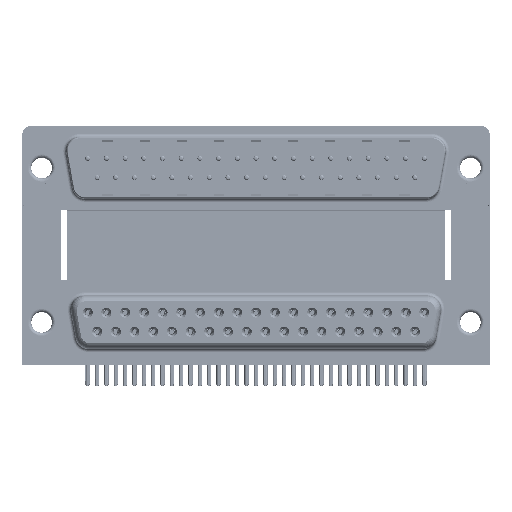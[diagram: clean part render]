
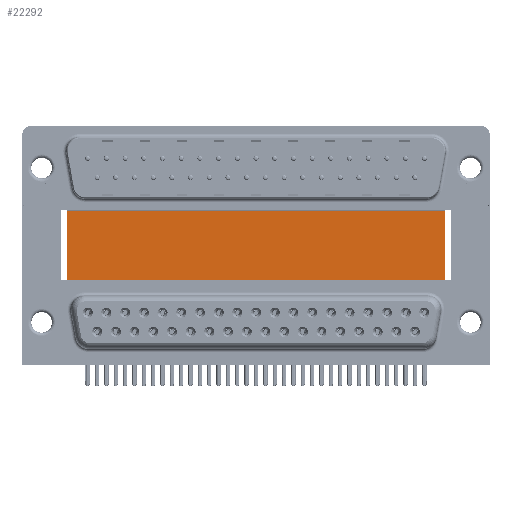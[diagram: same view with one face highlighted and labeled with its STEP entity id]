
A CAD part, top view. The second image highlights one B-rep face of the part: STEP entity #22292.
In plain terms, the highlighted planar face has unit normal (0, 0, 1).
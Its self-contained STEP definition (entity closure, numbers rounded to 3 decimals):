
#7515 = PLANE ( 'NONE',  #26577 ) ;
#13036 = CARTESIAN_POINT ( 'NONE',  ( 3.79, 16.585, -12. ) ) ;
#13248 = EDGE_CURVE ( 'NONE', #51506, #59921, #58317, .T. ) ;
#15172 = VECTOR ( 'NONE', #34135, 1000. ) ;
#16422 = ORIENTED_EDGE ( 'NONE', *, *, #55006, .T. ) ;
#18649 = EDGE_LOOP ( 'NONE', ( #16422, #38980, #28870, #19265 ) ) ;
#19265 = ORIENTED_EDGE ( 'NONE', *, *, #41314, .T. ) ;
#19292 = LINE ( 'NONE', #13036, #15172 ) ;
#22292 = ADVANCED_FACE ( 'NONE', ( #62328 ), #7515, .F. ) ;
#24802 = VECTOR ( 'NONE', #32882, 1000. ) ;
#26577 = AXIS2_PLACEMENT_3D ( 'NONE', #62976, #58341, #53389 ) ;
#26869 = CARTESIAN_POINT ( 'NONE',  ( 59.71, 16.585, -12. ) ) ;
#28870 = ORIENTED_EDGE ( 'NONE', *, *, #13248, .F. ) ;
#29016 = CARTESIAN_POINT ( 'NONE',  ( 3.79, -3.735, -12. ) ) ;
#31488 = LINE ( 'NONE', #26869, #51716 ) ;
#32882 = DIRECTION ( 'NONE',  ( 1., 0., 0. ) ) ;
#34135 = DIRECTION ( 'NONE',  ( 0., -1., 0. ) ) ;
#37174 = CARTESIAN_POINT ( 'NONE',  ( 59.71, 16.585, -12. ) ) ;
#37441 = EDGE_CURVE ( 'NONE', #59921, #44391, #31488, .T. ) ;
#38567 = CARTESIAN_POINT ( 'NONE',  ( 3.79, -3.735, -12. ) ) ;
#38980 = ORIENTED_EDGE ( 'NONE', *, *, #37441, .F. ) ;
#41314 = EDGE_CURVE ( 'NONE', #51506, #60748, #19292, .T. ) ;
#41406 = CARTESIAN_POINT ( 'NONE',  ( 3.79, 16.585, -12. ) ) ;
#42226 = VECTOR ( 'NONE', #64337, 1000. ) ;
#44391 = VERTEX_POINT ( 'NONE', #55547 ) ;
#46022 = DIRECTION ( 'NONE',  ( 0., -1., 0. ) ) ;
#51506 = VERTEX_POINT ( 'NONE', #41406 ) ;
#51716 = VECTOR ( 'NONE', #46022, 1000. ) ;
#53389 = DIRECTION ( 'NONE',  ( -1., 0., 0. ) ) ;
#54103 = LINE ( 'NONE', #29016, #42226 ) ;
#55006 = EDGE_CURVE ( 'NONE', #60748, #44391, #54103, .T. ) ;
#55547 = CARTESIAN_POINT ( 'NONE',  ( 59.71, -3.735, -12. ) ) ;
#58317 = LINE ( 'NONE', #62953, #24802 ) ;
#58341 = DIRECTION ( 'NONE',  ( 0., 0., -1. ) ) ;
#59921 = VERTEX_POINT ( 'NONE', #37174 ) ;
#60748 = VERTEX_POINT ( 'NONE', #38567 ) ;
#62328 = FACE_OUTER_BOUND ( 'NONE', #18649, .T. ) ;
#62953 = CARTESIAN_POINT ( 'NONE',  ( 3.79, 16.585, -12. ) ) ;
#62976 = CARTESIAN_POINT ( 'NONE',  ( 3.79, 16.585, -12. ) ) ;
#64337 = DIRECTION ( 'NONE',  ( 1., 0., 0. ) ) ;
